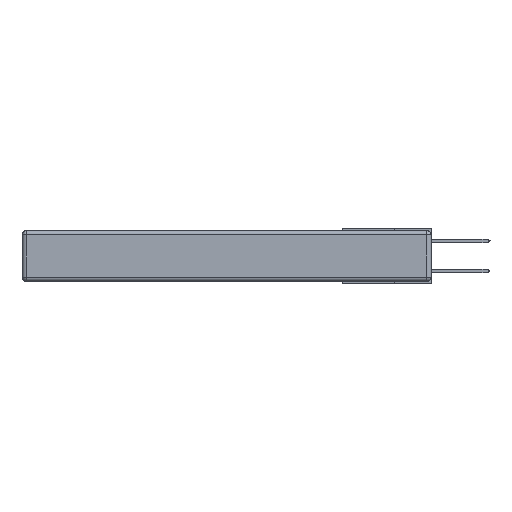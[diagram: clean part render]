
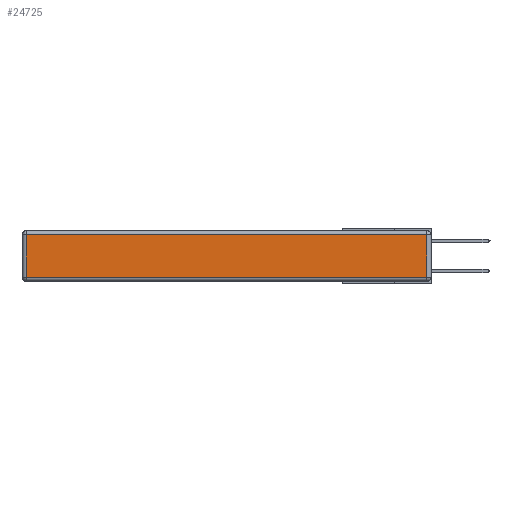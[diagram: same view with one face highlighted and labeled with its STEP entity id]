
A CAD part, left-side view. The second image highlights one B-rep face of the part: STEP entity #24725.
In plain terms, the highlighted planar face has unit normal (-1, 0, 0).
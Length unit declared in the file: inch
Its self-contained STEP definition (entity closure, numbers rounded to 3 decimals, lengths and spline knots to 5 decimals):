
#334 = CARTESIAN_POINT ( 'NONE',  ( 0., 0., -0.313 ) ) ;
#443 = EDGE_CURVE ( 'NONE', #2478, #2042, #19322, .T. ) ;
#1508 = CARTESIAN_POINT ( 'NONE',  ( 0., 0.03, -0.343 ) ) ;
#2042 = VERTEX_POINT ( 'NONE', #28569 ) ;
#2433 = EDGE_CURVE ( 'NONE', #10977, #27620, #22805, .T. ) ;
#2478 = VERTEX_POINT ( 'NONE', #14766 ) ;
#4648 = CARTESIAN_POINT ( 'NONE',  ( 0., 2.75, -0.03 ) ) ;
#5250 = DIRECTION ( 'NONE',  ( 0., 0., -1. ) ) ;
#5851 = DIRECTION ( 'NONE',  ( 0., 0., 1. ) ) ;
#5860 = ORIENTED_EDGE ( 'NONE', *, *, #443, .T. ) ;
#7036 = EDGE_CURVE ( 'NONE', #27620, #2478, #23269, .T. ) ;
#7312 = VECTOR ( 'NONE', #5851, 39.37008 ) ;
#7745 = CARTESIAN_POINT ( 'NONE',  ( 0., 2.72, -0.343 ) ) ;
#8533 = AXIS2_PLACEMENT_3D ( 'NONE', #9951, #12309, #26618 ) ;
#8708 = VECTOR ( 'NONE', #5250, 39.37008 ) ;
#8772 = LINE ( 'NONE', #1508, #7312 ) ;
#9951 = CARTESIAN_POINT ( 'NONE',  ( 0., 0., -0.343 ) ) ;
#10468 = VECTOR ( 'NONE', #28575, 39.37008 ) ;
#10977 = VERTEX_POINT ( 'NONE', #26739 ) ;
#12309 = DIRECTION ( 'NONE',  ( -1., 0., 0. ) ) ;
#14766 = CARTESIAN_POINT ( 'NONE',  ( 0., 2.72, -0.313 ) ) ;
#17034 = FACE_OUTER_BOUND ( 'NONE', #23502, .T. ) ;
#19322 = LINE ( 'NONE', #334, #21511 ) ;
#20119 = ORIENTED_EDGE ( 'NONE', *, *, #2433, .T. ) ;
#20652 = ORIENTED_EDGE ( 'NONE', *, *, #7036, .T. ) ;
#21511 = VECTOR ( 'NONE', #23410, 39.37008 ) ;
#22377 = CARTESIAN_POINT ( 'NONE',  ( 0., 2.72, -0.03 ) ) ;
#22423 = ORIENTED_EDGE ( 'NONE', *, *, #28744, .T. ) ;
#22805 = LINE ( 'NONE', #4648, #10468 ) ;
#23269 = LINE ( 'NONE', #7745, #8708 ) ;
#23410 = DIRECTION ( 'NONE',  ( 0., -1., 0. ) ) ;
#23502 = EDGE_LOOP ( 'NONE', ( #5860, #22423, #20119, #20652 ) ) ;
#23776 = PLANE ( 'NONE',  #8533 ) ;
#24725 = ADVANCED_FACE ( 'NONE', ( #17034 ), #23776, .T. ) ;
#26618 = DIRECTION ( 'NONE',  ( 0., 0., 1. ) ) ;
#26739 = CARTESIAN_POINT ( 'NONE',  ( 0., 0.03, -0.03 ) ) ;
#27620 = VERTEX_POINT ( 'NONE', #22377 ) ;
#28569 = CARTESIAN_POINT ( 'NONE',  ( 0., 0.03, -0.313 ) ) ;
#28575 = DIRECTION ( 'NONE',  ( 0., 1., 0. ) ) ;
#28744 = EDGE_CURVE ( 'NONE', #2042, #10977, #8772, .T. ) ;
